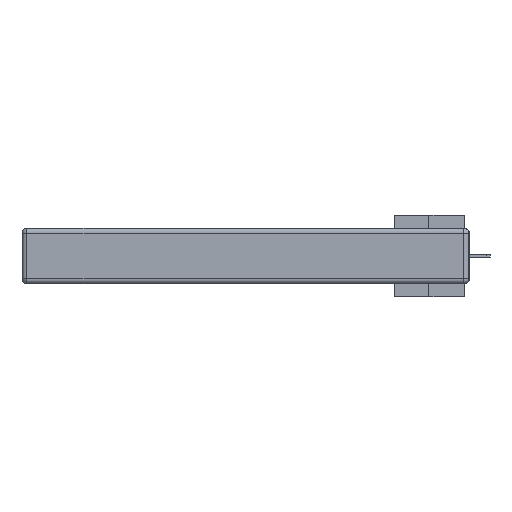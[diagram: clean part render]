
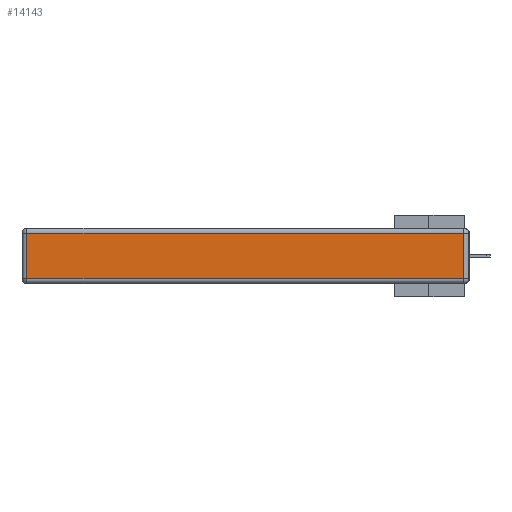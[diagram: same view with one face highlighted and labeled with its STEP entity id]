
A CAD part, left-side view. The second image highlights one B-rep face of the part: STEP entity #14143.
In plain terms, the highlighted planar face has unit normal (-1, 0, 0).
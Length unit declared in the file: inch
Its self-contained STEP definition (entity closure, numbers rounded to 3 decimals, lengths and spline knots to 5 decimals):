
#1282 = DIRECTION ( 'NONE',  ( 0., 1., 0. ) ) ;
#2048 = VECTOR ( 'NONE', #12989, 39.37008 ) ;
#2952 = ORIENTED_EDGE ( 'NONE', *, *, #8720, .T. ) ;
#3328 = CARTESIAN_POINT ( 'NONE',  ( 0., 2.72, -0.343 ) ) ;
#3630 = EDGE_CURVE ( 'NONE', #25046, #6372, #27714, .T. ) ;
#6372 = VERTEX_POINT ( 'NONE', #8712 ) ;
#7081 = AXIS2_PLACEMENT_3D ( 'NONE', #22518, #15568, #17915 ) ;
#8226 = CARTESIAN_POINT ( 'NONE',  ( 0., 0.03, -0.03 ) ) ;
#8712 = CARTESIAN_POINT ( 'NONE',  ( 0., 2.72, -0.03 ) ) ;
#8720 = EDGE_CURVE ( 'NONE', #21381, #23688, #30642, .T. ) ;
#8837 = CARTESIAN_POINT ( 'NONE',  ( 0., 2.75, -0.03 ) ) ;
#10773 = CARTESIAN_POINT ( 'NONE',  ( 0., 2.72, -0.313 ) ) ;
#11147 = VECTOR ( 'NONE', #14352, 39.37008 ) ;
#12989 = DIRECTION ( 'NONE',  ( 0., 0., -1. ) ) ;
#14143 = ADVANCED_FACE ( 'NONE', ( #21043 ), #29366, .T. ) ;
#14352 = DIRECTION ( 'NONE',  ( 0., 0., 1. ) ) ;
#15039 = EDGE_LOOP ( 'NONE', ( #2952, #17807, #16360, #21553 ) ) ;
#15568 = DIRECTION ( 'NONE',  ( -1., 0., 0. ) ) ;
#16360 = ORIENTED_EDGE ( 'NONE', *, *, #3630, .T. ) ;
#17237 = VECTOR ( 'NONE', #1282, 39.37008 ) ;
#17807 = ORIENTED_EDGE ( 'NONE', *, *, #28369, .T. ) ;
#17915 = DIRECTION ( 'NONE',  ( 0., 0., 1. ) ) ;
#19183 = EDGE_CURVE ( 'NONE', #6372, #21381, #21987, .T. ) ;
#20881 = DIRECTION ( 'NONE',  ( 0., -1., 0. ) ) ;
#21043 = FACE_OUTER_BOUND ( 'NONE', #15039, .T. ) ;
#21381 = VERTEX_POINT ( 'NONE', #10773 ) ;
#21553 = ORIENTED_EDGE ( 'NONE', *, *, #19183, .T. ) ;
#21987 = LINE ( 'NONE', #3328, #2048 ) ;
#22518 = CARTESIAN_POINT ( 'NONE',  ( 0., 0., -0.343 ) ) ;
#23688 = VERTEX_POINT ( 'NONE', #27140 ) ;
#25046 = VERTEX_POINT ( 'NONE', #8226 ) ;
#25960 = CARTESIAN_POINT ( 'NONE',  ( 0., 0., -0.313 ) ) ;
#26289 = CARTESIAN_POINT ( 'NONE',  ( 0., 0.03, -0.343 ) ) ;
#27140 = CARTESIAN_POINT ( 'NONE',  ( 0., 0.03, -0.313 ) ) ;
#27714 = LINE ( 'NONE', #8837, #17237 ) ;
#28369 = EDGE_CURVE ( 'NONE', #23688, #25046, #29980, .T. ) ;
#29366 = PLANE ( 'NONE',  #7081 ) ;
#29533 = VECTOR ( 'NONE', #20881, 39.37008 ) ;
#29980 = LINE ( 'NONE', #26289, #11147 ) ;
#30642 = LINE ( 'NONE', #25960, #29533 ) ;
